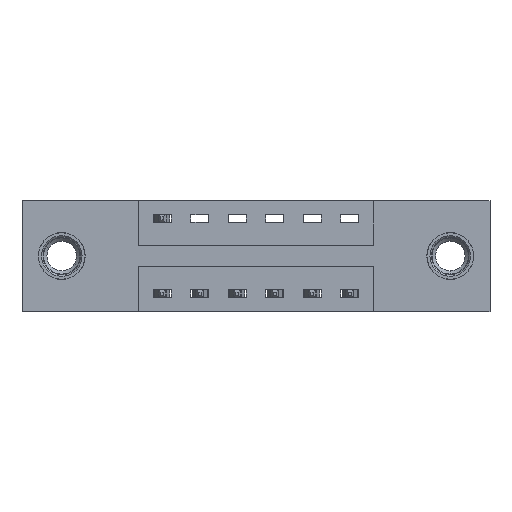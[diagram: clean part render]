
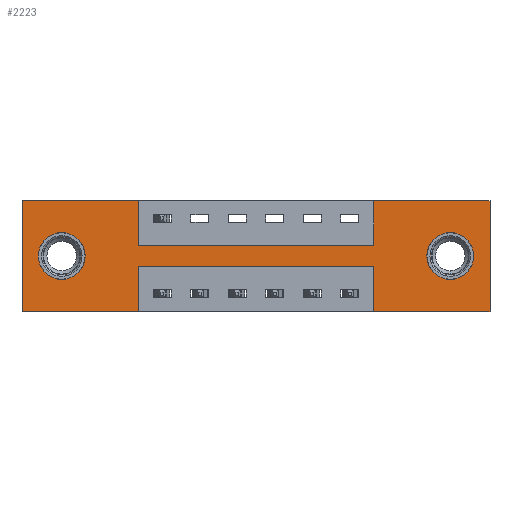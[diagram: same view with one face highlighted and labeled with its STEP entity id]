
A CAD part, front view. The second image highlights one B-rep face of the part: STEP entity #2223.
In plain terms, the highlighted planar face has unit normal (0, -1, 0).
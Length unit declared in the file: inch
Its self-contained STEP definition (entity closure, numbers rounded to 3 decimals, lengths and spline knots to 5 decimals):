
#119 = DIRECTION ( 'NONE',  ( 0., 0., -1. ) ) ;
#190 = ORIENTED_EDGE ( 'NONE', *, *, #6084, .F. ) ;
#226 = LINE ( 'NONE', #5783, #3863 ) ;
#240 = CARTESIAN_POINT ( 'NONE',  ( 1.4275, 0., -0.107 ) ) ;
#303 = CARTESIAN_POINT ( 'NONE',  ( 0.3875, 0., -0.37 ) ) ;
#398 = VERTEX_POINT ( 'NONE', #706 ) ;
#697 = CARTESIAN_POINT ( 'NONE',  ( 0.3875, 0., -0.15 ) ) ;
#699 = VERTEX_POINT ( 'NONE', #240 ) ;
#705 = EDGE_CURVE ( 'NONE', #7408, #4146, #2315, .T. ) ;
#706 = CARTESIAN_POINT ( 'NONE',  ( 1.4275, 0., -0.263 ) ) ;
#760 = EDGE_LOOP ( 'NONE', ( #6051, #8433, #190, #9554, #4431, #1719, #8222, #812, #3831, #6725, #5578, #6738 ) ) ;
#812 = ORIENTED_EDGE ( 'NONE', *, *, #2831, .F. ) ;
#853 = VECTOR ( 'NONE', #3332, 39.37008 ) ;
#873 = VECTOR ( 'NONE', #9128, 39.37008 ) ;
#891 = EDGE_CURVE ( 'NONE', #5468, #6721, #1123, .T. ) ;
#1123 = CIRCLE ( 'NONE', #9525, 0.078 ) ;
#1264 = VERTEX_POINT ( 'NONE', #4360 ) ;
#1371 = EDGE_CURVE ( 'NONE', #1264, #6395, #3169, .T. ) ;
#1391 = EDGE_CURVE ( 'NONE', #6831, #8248, #8648, .T. ) ;
#1573 = CARTESIAN_POINT ( 'NONE',  ( 0., 0., 0. ) ) ;
#1719 = ORIENTED_EDGE ( 'NONE', *, *, #5675, .F. ) ;
#1723 = CIRCLE ( 'NONE', #9133, 0.078 ) ;
#1792 = DIRECTION ( 'NONE',  ( 0., 1., 0. ) ) ;
#2111 = FACE_OUTER_BOUND ( 'NONE', #760, .T. ) ;
#2181 = EDGE_CURVE ( 'NONE', #8057, #3148, #4603, .T. ) ;
#2189 = VERTEX_POINT ( 'NONE', #6083 ) ;
#2223 = ADVANCED_FACE ( 'NONE', ( #8336, #4125, #2111 ), #5590, .T. ) ;
#2315 = LINE ( 'NONE', #303, #6338 ) ;
#2613 = ORIENTED_EDGE ( 'NONE', *, *, #891, .T. ) ;
#2676 = VECTOR ( 'NONE', #9226, 39.37008 ) ;
#2738 = VECTOR ( 'NONE', #8533, 39.37008 ) ;
#2831 = EDGE_CURVE ( 'NONE', #9828, #8057, #2931, .T. ) ;
#2930 = EDGE_CURVE ( 'NONE', #2189, #7408, #5764, .T. ) ;
#2931 = LINE ( 'NONE', #9091, #873 ) ;
#2938 = VERTEX_POINT ( 'NONE', #8524 ) ;
#2974 = EDGE_CURVE ( 'NONE', #4146, #1264, #5991, .T. ) ;
#3053 = CARTESIAN_POINT ( 'NONE',  ( 0.3875, 0., -0.37 ) ) ;
#3148 = VERTEX_POINT ( 'NONE', #8009 ) ;
#3169 = LINE ( 'NONE', #1573, #853 ) ;
#3295 = DIRECTION ( 'NONE',  ( 0., 1., 0. ) ) ;
#3312 = VERTEX_POINT ( 'NONE', #6949 ) ;
#3332 = DIRECTION ( 'NONE',  ( 0., 0., 1. ) ) ;
#3472 = EDGE_CURVE ( 'NONE', #2938, #9828, #8306, .T. ) ;
#3549 = EDGE_CURVE ( 'NONE', #6395, #2938, #226, .T. ) ;
#3561 = LINE ( 'NONE', #4101, #5326 ) ;
#3710 = ORIENTED_EDGE ( 'NONE', *, *, #9621, .T. ) ;
#3765 = VECTOR ( 'NONE', #8561, 39.37008 ) ;
#3826 = CARTESIAN_POINT ( 'NONE',  ( 0., 0., 0. ) ) ;
#3831 = ORIENTED_EDGE ( 'NONE', *, *, #3472, .F. ) ;
#3863 = VECTOR ( 'NONE', #5813, 39.37008 ) ;
#3983 = CIRCLE ( 'NONE', #8951, 0.078 ) ;
#4080 = DIRECTION ( 'NONE',  ( 0., 1., 0. ) ) ;
#4095 = CARTESIAN_POINT ( 'NONE',  ( 0.1325, 0., -0.185 ) ) ;
#4101 = CARTESIAN_POINT ( 'NONE',  ( 0., 0., -0.37 ) ) ;
#4125 = FACE_BOUND ( 'NONE', #8569, .T. ) ;
#4146 = VERTEX_POINT ( 'NONE', #3053 ) ;
#4173 = DIRECTION ( 'NONE',  ( 0., 0., 1. ) ) ;
#4307 = CARTESIAN_POINT ( 'NONE',  ( 0.1325, 0., -0.185 ) ) ;
#4360 = CARTESIAN_POINT ( 'NONE',  ( 0., 0., -0.37 ) ) ;
#4431 = ORIENTED_EDGE ( 'NONE', *, *, #1391, .F. ) ;
#4517 = VECTOR ( 'NONE', #5111, 39.37008 ) ;
#4603 = LINE ( 'NONE', #6104, #6583 ) ;
#4845 = EDGE_LOOP ( 'NONE', ( #7421, #5636 ) ) ;
#4939 = CARTESIAN_POINT ( 'NONE',  ( 0.1325, 0., -0.263 ) ) ;
#5063 = DIRECTION ( 'NONE',  ( 0., 0., 1. ) ) ;
#5111 = DIRECTION ( 'NONE',  ( 1., 0., 0. ) ) ;
#5326 = VECTOR ( 'NONE', #6360, 39.37008 ) ;
#5379 = DIRECTION ( 'NONE',  ( 0., 0., -1. ) ) ;
#5421 = DIRECTION ( 'NONE',  ( 0., -1., 0. ) ) ;
#5468 = VERTEX_POINT ( 'NONE', #6357 ) ;
#5578 = ORIENTED_EDGE ( 'NONE', *, *, #1371, .F. ) ;
#5590 = PLANE ( 'NONE',  #9097 ) ;
#5636 = ORIENTED_EDGE ( 'NONE', *, *, #7242, .T. ) ;
#5675 = EDGE_CURVE ( 'NONE', #3148, #6831, #6510, .T. ) ;
#5703 = CARTESIAN_POINT ( 'NONE',  ( 0., 0., -0.37 ) ) ;
#5764 = LINE ( 'NONE', #8606, #3765 ) ;
#5783 = CARTESIAN_POINT ( 'NONE',  ( 0., 0., 0. ) ) ;
#5813 = DIRECTION ( 'NONE',  ( 1., 0., 0. ) ) ;
#5991 = LINE ( 'NONE', #8498, #9256 ) ;
#6028 = CIRCLE ( 'NONE', #8106, 0.078 ) ;
#6051 = ORIENTED_EDGE ( 'NONE', *, *, #705, .F. ) ;
#6083 = CARTESIAN_POINT ( 'NONE',  ( 1.1725, 0., -0.22 ) ) ;
#6084 = EDGE_CURVE ( 'NONE', #3312, #2189, #6730, .T. ) ;
#6092 = DIRECTION ( 'NONE',  ( 0., 0., -1. ) ) ;
#6104 = CARTESIAN_POINT ( 'NONE',  ( 1.1725, 0., 0. ) ) ;
#6149 = CARTESIAN_POINT ( 'NONE',  ( 0.3875, 0., 0. ) ) ;
#6236 = DIRECTION ( 'NONE',  ( 0., 0., 1. ) ) ;
#6294 = CARTESIAN_POINT ( 'NONE',  ( 1.4275, 0., -0.185 ) ) ;
#6324 = VECTOR ( 'NONE', #6092, 39.37008 ) ;
#6338 = VECTOR ( 'NONE', #119, 39.37008 ) ;
#6357 = CARTESIAN_POINT ( 'NONE',  ( 0.1325, 0., -0.107 ) ) ;
#6360 = DIRECTION ( 'NONE',  ( -1., 0., 0. ) ) ;
#6395 = VERTEX_POINT ( 'NONE', #3826 ) ;
#6510 = LINE ( 'NONE', #8071, #4517 ) ;
#6583 = VECTOR ( 'NONE', #6236, 39.37008 ) ;
#6721 = VERTEX_POINT ( 'NONE', #4939 ) ;
#6725 = ORIENTED_EDGE ( 'NONE', *, *, #3549, .F. ) ;
#6730 = LINE ( 'NONE', #7760, #2738 ) ;
#6738 = ORIENTED_EDGE ( 'NONE', *, *, #2974, .F. ) ;
#6831 = VERTEX_POINT ( 'NONE', #9540 ) ;
#6949 = CARTESIAN_POINT ( 'NONE',  ( 1.1725, 0., -0.37 ) ) ;
#7044 = DIRECTION ( 'NONE',  ( 0., 0., -1. ) ) ;
#7207 = CARTESIAN_POINT ( 'NONE',  ( 0.3875, 0., -0.22 ) ) ;
#7242 = EDGE_CURVE ( 'NONE', #398, #699, #6028, .T. ) ;
#7298 = EDGE_CURVE ( 'NONE', #8248, #3312, #3561, .T. ) ;
#7408 = VERTEX_POINT ( 'NONE', #7207 ) ;
#7421 = ORIENTED_EDGE ( 'NONE', *, *, #9386, .T. ) ;
#7752 = CARTESIAN_POINT ( 'NONE',  ( 1.4275, 0., -0.185 ) ) ;
#7760 = CARTESIAN_POINT ( 'NONE',  ( 1.1725, 0., -0.37 ) ) ;
#8009 = CARTESIAN_POINT ( 'NONE',  ( 1.1725, 0., 0. ) ) ;
#8057 = VERTEX_POINT ( 'NONE', #8411 ) ;
#8071 = CARTESIAN_POINT ( 'NONE',  ( 0., 0., 0. ) ) ;
#8106 = AXIS2_PLACEMENT_3D ( 'NONE', #6294, #1792, #7044 ) ;
#8222 = ORIENTED_EDGE ( 'NONE', *, *, #2181, .F. ) ;
#8248 = VERTEX_POINT ( 'NONE', #8633 ) ;
#8306 = LINE ( 'NONE', #6149, #6324 ) ;
#8336 = FACE_BOUND ( 'NONE', #4845, .T. ) ;
#8411 = CARTESIAN_POINT ( 'NONE',  ( 1.1725, 0., -0.15 ) ) ;
#8433 = ORIENTED_EDGE ( 'NONE', *, *, #2930, .F. ) ;
#8453 = DIRECTION ( 'NONE',  ( -1., 0., 0. ) ) ;
#8498 = CARTESIAN_POINT ( 'NONE',  ( 0., 0., -0.37 ) ) ;
#8521 = DIRECTION ( 'NONE',  ( 0., 0., -1. ) ) ;
#8524 = CARTESIAN_POINT ( 'NONE',  ( 0.3875, 0., 0. ) ) ;
#8533 = DIRECTION ( 'NONE',  ( 0., 0., 1. ) ) ;
#8561 = DIRECTION ( 'NONE',  ( -1., 0., 0. ) ) ;
#8569 = EDGE_LOOP ( 'NONE', ( #2613, #3710 ) ) ;
#8606 = CARTESIAN_POINT ( 'NONE',  ( 0.3875, 0., -0.22 ) ) ;
#8633 = CARTESIAN_POINT ( 'NONE',  ( 1.56, 0., -0.37 ) ) ;
#8648 = LINE ( 'NONE', #9443, #2676 ) ;
#8951 = AXIS2_PLACEMENT_3D ( 'NONE', #4307, #9535, #5063 ) ;
#9091 = CARTESIAN_POINT ( 'NONE',  ( 0.3875, 0., -0.15 ) ) ;
#9097 = AXIS2_PLACEMENT_3D ( 'NONE', #5703, #5421, #5379 ) ;
#9128 = DIRECTION ( 'NONE',  ( 1., 0., 0. ) ) ;
#9133 = AXIS2_PLACEMENT_3D ( 'NONE', #7752, #3295, #8521 ) ;
#9226 = DIRECTION ( 'NONE',  ( 0., 0., -1. ) ) ;
#9256 = VECTOR ( 'NONE', #8453, 39.37008 ) ;
#9386 = EDGE_CURVE ( 'NONE', #699, #398, #1723, .T. ) ;
#9443 = CARTESIAN_POINT ( 'NONE',  ( 1.56, 0., 0. ) ) ;
#9525 = AXIS2_PLACEMENT_3D ( 'NONE', #4095, #4080, #4173 ) ;
#9535 = DIRECTION ( 'NONE',  ( 0., 1., 0. ) ) ;
#9540 = CARTESIAN_POINT ( 'NONE',  ( 1.56, 0., 0. ) ) ;
#9554 = ORIENTED_EDGE ( 'NONE', *, *, #7298, .F. ) ;
#9621 = EDGE_CURVE ( 'NONE', #6721, #5468, #3983, .T. ) ;
#9828 = VERTEX_POINT ( 'NONE', #697 ) ;
